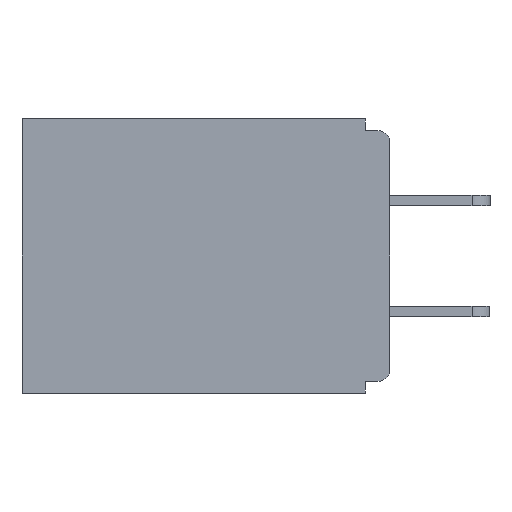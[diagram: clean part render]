
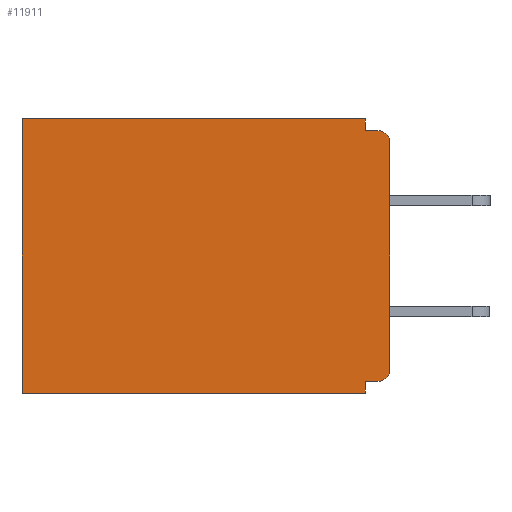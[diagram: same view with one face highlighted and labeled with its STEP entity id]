
A CAD part, left-side view. The second image highlights one B-rep face of the part: STEP entity #11911.
In plain terms, the highlighted planar face has unit normal (-1, 0, 0).
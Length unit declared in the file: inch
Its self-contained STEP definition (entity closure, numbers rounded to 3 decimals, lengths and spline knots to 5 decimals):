
#41 = VECTOR ( 'NONE', #13491, 39.37008 ) ;
#64 = CIRCLE ( 'NONE', #13403, 0.015 ) ;
#504 = DIRECTION ( 'NONE',  ( 0., 0., -1. ) ) ;
#525 = ORIENTED_EDGE ( 'NONE', *, *, #2311, .T. ) ;
#582 = ORIENTED_EDGE ( 'NONE', *, *, #7961, .T. ) ;
#790 = LINE ( 'NONE', #1987, #4894 ) ;
#801 = DIRECTION ( 'NONE',  ( 0., 0., -1. ) ) ;
#975 = VECTOR ( 'NONE', #3548, 39.37008 ) ;
#1049 = EDGE_CURVE ( 'NONE', #12591, #1314, #790, .T. ) ;
#1109 = CARTESIAN_POINT ( 'NONE',  ( 0.298, 0., -0.03 ) ) ;
#1178 = VERTEX_POINT ( 'NONE', #8302 ) ;
#1187 = CARTESIAN_POINT ( 'NONE',  ( 0.298, 0., -0.313 ) ) ;
#1202 = CARTESIAN_POINT ( 'NONE',  ( 0.298, 0.031, -0.015 ) ) ;
#1282 = ORIENTED_EDGE ( 'NONE', *, *, #1049, .F. ) ;
#1314 = VERTEX_POINT ( 'NONE', #12721 ) ;
#1752 = DIRECTION ( 'NONE',  ( -1., 0., 0. ) ) ;
#1834 = CARTESIAN_POINT ( 'NONE',  ( 0.298, 0.46, 0. ) ) ;
#1884 = DIRECTION ( 'NONE',  ( 0., 0., -1. ) ) ;
#1987 = CARTESIAN_POINT ( 'NONE',  ( 0.298, 0.031, -0.343 ) ) ;
#2047 = CARTESIAN_POINT ( 'NONE',  ( 0.298, 0.015, -0.015 ) ) ;
#2224 = ORIENTED_EDGE ( 'NONE', *, *, #5993, .F. ) ;
#2311 = EDGE_CURVE ( 'NONE', #11190, #5784, #64, .T. ) ;
#2374 = CARTESIAN_POINT ( 'NONE',  ( 0.298, 0.031, -0.343 ) ) ;
#2509 = DIRECTION ( 'NONE',  ( 0., 0., -1. ) ) ;
#3330 = VERTEX_POINT ( 'NONE', #5798 ) ;
#3355 = AXIS2_PLACEMENT_3D ( 'NONE', #13032, #7442, #1884 ) ;
#3418 = CARTESIAN_POINT ( 'NONE',  ( 0.298, 0., 0. ) ) ;
#3548 = DIRECTION ( 'NONE',  ( 0., 1., 0. ) ) ;
#3784 = CARTESIAN_POINT ( 'NONE',  ( 0.298, 0., -0.328 ) ) ;
#3884 = DIRECTION ( 'NONE',  ( 0., 1., 0. ) ) ;
#4788 = ORIENTED_EDGE ( 'NONE', *, *, #9517, .F. ) ;
#4894 = VECTOR ( 'NONE', #9759, 39.37008 ) ;
#5030 = CARTESIAN_POINT ( 'NONE',  ( 0.298, 0.46, 0. ) ) ;
#5400 = EDGE_CURVE ( 'NONE', #1314, #3330, #8249, .T. ) ;
#5784 = VERTEX_POINT ( 'NONE', #2047 ) ;
#5798 = CARTESIAN_POINT ( 'NONE',  ( 0.298, 0.46, -0.343 ) ) ;
#5833 = VERTEX_POINT ( 'NONE', #1187 ) ;
#5993 = EDGE_CURVE ( 'NONE', #6598, #11654, #9265, .T. ) ;
#6262 = FACE_OUTER_BOUND ( 'NONE', #11234, .T. ) ;
#6598 = VERTEX_POINT ( 'NONE', #7567 ) ;
#6724 = CARTESIAN_POINT ( 'NONE',  ( 0.298, 0.015, -0.313 ) ) ;
#6841 = DIRECTION ( 'NONE',  ( 0., -1., 0. ) ) ;
#7280 = EDGE_CURVE ( 'NONE', #11190, #5833, #8386, .T. ) ;
#7442 = DIRECTION ( 'NONE',  ( 1., 0., 0. ) ) ;
#7567 = CARTESIAN_POINT ( 'NONE',  ( 0.298, 0.031, 0. ) ) ;
#7656 = ORIENTED_EDGE ( 'NONE', *, *, #7280, .F. ) ;
#7808 = ORIENTED_EDGE ( 'NONE', *, *, #11745, .T. ) ;
#7867 = VECTOR ( 'NONE', #801, 39.37008 ) ;
#7961 = EDGE_CURVE ( 'NONE', #6598, #13360, #13531, .T. ) ;
#8017 = CARTESIAN_POINT ( 'NONE',  ( 0.298, 0., -0.015 ) ) ;
#8021 = EDGE_CURVE ( 'NONE', #1178, #5833, #11145, .T. ) ;
#8133 = DIRECTION ( 'NONE',  ( -1., 0., 0. ) ) ;
#8249 = LINE ( 'NONE', #10169, #975 ) ;
#8302 = CARTESIAN_POINT ( 'NONE',  ( 0.298, 0.015, -0.328 ) ) ;
#8386 = LINE ( 'NONE', #14042, #7867 ) ;
#8398 = LINE ( 'NONE', #8017, #10458 ) ;
#8423 = CARTESIAN_POINT ( 'NONE',  ( 0.298, 0.015, -0.03 ) ) ;
#9026 = ORIENTED_EDGE ( 'NONE', *, *, #5400, .F. ) ;
#9265 = LINE ( 'NONE', #2374, #10864 ) ;
#9451 = AXIS2_PLACEMENT_3D ( 'NONE', #6724, #8133, #13607 ) ;
#9517 = EDGE_CURVE ( 'NONE', #1178, #12591, #13623, .T. ) ;
#9759 = DIRECTION ( 'NONE',  ( 0., 0., -1. ) ) ;
#9983 = ORIENTED_EDGE ( 'NONE', *, *, #10542, .F. ) ;
#10169 = CARTESIAN_POINT ( 'NONE',  ( 0.298, 0., -0.343 ) ) ;
#10458 = VECTOR ( 'NONE', #6841, 39.37008 ) ;
#10542 = EDGE_CURVE ( 'NONE', #11654, #5784, #8398, .T. ) ;
#10864 = VECTOR ( 'NONE', #2509, 39.37008 ) ;
#10951 = LINE ( 'NONE', #5030, #14224 ) ;
#11145 = CIRCLE ( 'NONE', #9451, 0.015 ) ;
#11190 = VERTEX_POINT ( 'NONE', #1109 ) ;
#11234 = EDGE_LOOP ( 'NONE', ( #525, #9983, #2224, #582, #7808, #9026, #1282, #4788, #12064, #7656 ) ) ;
#11654 = VERTEX_POINT ( 'NONE', #1202 ) ;
#11745 = EDGE_CURVE ( 'NONE', #13360, #3330, #10951, .T. ) ;
#11911 = ADVANCED_FACE ( 'NONE', ( #6262 ), #11951, .F. ) ;
#11951 = PLANE ( 'NONE',  #3355 ) ;
#11961 = DIRECTION ( 'NONE',  ( 0., 0., -1. ) ) ;
#12064 = ORIENTED_EDGE ( 'NONE', *, *, #8021, .T. ) ;
#12512 = CARTESIAN_POINT ( 'NONE',  ( 0.298, 0.031, -0.328 ) ) ;
#12591 = VERTEX_POINT ( 'NONE', #12512 ) ;
#12721 = CARTESIAN_POINT ( 'NONE',  ( 0.298, 0.031, -0.343 ) ) ;
#13032 = CARTESIAN_POINT ( 'NONE',  ( 0.298, 0., 0. ) ) ;
#13360 = VERTEX_POINT ( 'NONE', #1834 ) ;
#13403 = AXIS2_PLACEMENT_3D ( 'NONE', #8423, #1752, #11961 ) ;
#13491 = DIRECTION ( 'NONE',  ( 0., 1., 0. ) ) ;
#13531 = LINE ( 'NONE', #3418, #41 ) ;
#13607 = DIRECTION ( 'NONE',  ( 0., 0., -1. ) ) ;
#13623 = LINE ( 'NONE', #3784, #14186 ) ;
#14042 = CARTESIAN_POINT ( 'NONE',  ( 0.298, 0., 0. ) ) ;
#14186 = VECTOR ( 'NONE', #3884, 39.37008 ) ;
#14224 = VECTOR ( 'NONE', #504, 39.37008 ) ;
